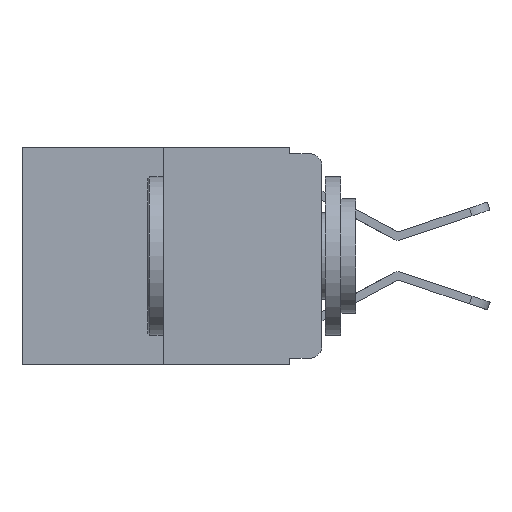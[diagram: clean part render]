
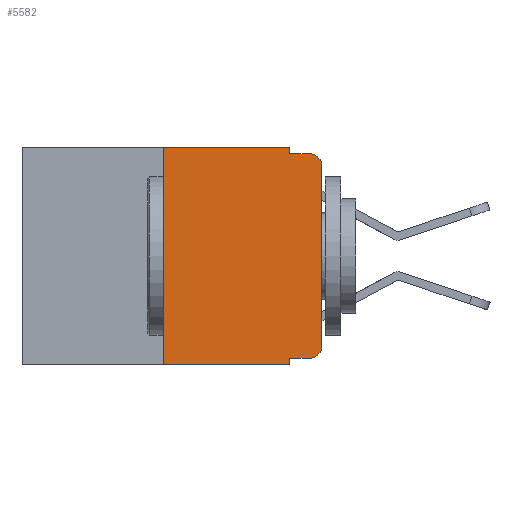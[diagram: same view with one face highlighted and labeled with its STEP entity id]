
A CAD part, left-side view. The second image highlights one B-rep face of the part: STEP entity #5582.
In plain terms, the highlighted planar face has unit normal (-1, 0, 0).
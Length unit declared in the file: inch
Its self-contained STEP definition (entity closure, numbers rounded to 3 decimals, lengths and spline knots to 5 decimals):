
#95 = VERTEX_POINT ( 'NONE', #556 ) ;
#371 = DIRECTION ( 'NONE',  ( 0., 0., 1. ) ) ;
#556 = CARTESIAN_POINT ( 'NONE',  ( 0., 0.051, -0.343 ) ) ;
#577 = EDGE_CURVE ( 'NONE', #708, #95, #7618, .T. ) ;
#708 = VERTEX_POINT ( 'NONE', #16838 ) ;
#1012 = LINE ( 'NONE', #12679, #2255 ) ;
#1242 = VERTEX_POINT ( 'NONE', #6102 ) ;
#1489 = VERTEX_POINT ( 'NONE', #12013 ) ;
#2255 = VECTOR ( 'NONE', #16822, 39.37008 ) ;
#2292 = EDGE_CURVE ( 'NONE', #1242, #5987, #1012, .T. ) ;
#2362 = EDGE_LOOP ( 'NONE', ( #12966, #10455, #10580, #13551, #6723, #7793, #7699, #6070, #3460, #5937 ) ) ;
#2534 = LINE ( 'NONE', #16949, #16936 ) ;
#2572 = DIRECTION ( 'NONE',  ( 0., -1., 0. ) ) ;
#3074 = VECTOR ( 'NONE', #4024, 39.37008 ) ;
#3460 = ORIENTED_EDGE ( 'NONE', *, *, #13911, .T. ) ;
#3461 = EDGE_CURVE ( 'NONE', #708, #11666, #15103, .T. ) ;
#4012 = DIRECTION ( 'NONE',  ( -1., 0., 0. ) ) ;
#4024 = DIRECTION ( 'NONE',  ( 0., 0., -1. ) ) ;
#4163 = DIRECTION ( 'NONE',  ( 0., -1., 0. ) ) ;
#4422 = CARTESIAN_POINT ( 'NONE',  ( 0., 0., 0. ) ) ;
#4485 = VERTEX_POINT ( 'NONE', #6245 ) ;
#4686 = EDGE_CURVE ( 'NONE', #11666, #1242, #9004, .T. ) ;
#5286 = DIRECTION ( 'NONE',  ( 1., 0., 0. ) ) ;
#5328 = CARTESIAN_POINT ( 'NONE',  ( 0., 0.02, -0.313 ) ) ;
#5380 = FACE_OUTER_BOUND ( 'NONE', #2362, .T. ) ;
#5458 = CARTESIAN_POINT ( 'NONE',  ( 0., 0.051, 0. ) ) ;
#5460 = PLANE ( 'NONE',  #8313 ) ;
#5499 = DIRECTION ( 'NONE',  ( 0., 0., -1. ) ) ;
#5582 = ADVANCED_FACE ( 'NONE', ( #5380 ), #5460, .F. ) ;
#5701 = LINE ( 'NONE', #7719, #11393 ) ;
#5756 = CARTESIAN_POINT ( 'NONE',  ( 0., 0.02, -0.01 ) ) ;
#5937 = ORIENTED_EDGE ( 'NONE', *, *, #6556, .T. ) ;
#5987 = VERTEX_POINT ( 'NONE', #14059 ) ;
#6070 = ORIENTED_EDGE ( 'NONE', *, *, #15875, .F. ) ;
#6102 = CARTESIAN_POINT ( 'NONE',  ( 0., 0.051, 0. ) ) ;
#6245 = CARTESIAN_POINT ( 'NONE',  ( 0., 0.02, -0.333 ) ) ;
#6556 = EDGE_CURVE ( 'NONE', #4485, #11104, #9183, .T. ) ;
#6686 = VECTOR ( 'NONE', #371, 39.37008 ) ;
#6723 = ORIENTED_EDGE ( 'NONE', *, *, #4686, .F. ) ;
#6859 = DIRECTION ( 'NONE',  ( -1., 0., 0. ) ) ;
#7618 = LINE ( 'NONE', #8434, #13956 ) ;
#7699 = ORIENTED_EDGE ( 'NONE', *, *, #577, .T. ) ;
#7719 = CARTESIAN_POINT ( 'NONE',  ( 0., 0.051, -0.333 ) ) ;
#7793 = ORIENTED_EDGE ( 'NONE', *, *, #3461, .F. ) ;
#7939 = VERTEX_POINT ( 'NONE', #5756 ) ;
#8172 = DIRECTION ( 'NONE',  ( 0., 0., -1. ) ) ;
#8313 = AXIS2_PLACEMENT_3D ( 'NONE', #9300, #5286, #8172 ) ;
#8434 = CARTESIAN_POINT ( 'NONE',  ( 0., 0.473, -0.343 ) ) ;
#9004 = LINE ( 'NONE', #10656, #13454 ) ;
#9183 = CIRCLE ( 'NONE', #13985, 0.02 ) ;
#9300 = CARTESIAN_POINT ( 'NONE',  ( 0., 0.473, 0. ) ) ;
#9343 = EDGE_CURVE ( 'NONE', #5987, #7939, #2534, .T. ) ;
#10279 = CARTESIAN_POINT ( 'NONE',  ( 0., 0.25, 0. ) ) ;
#10343 = DIRECTION ( 'NONE',  ( 0., -1., 0. ) ) ;
#10455 = ORIENTED_EDGE ( 'NONE', *, *, #16005, .T. ) ;
#10580 = ORIENTED_EDGE ( 'NONE', *, *, #9343, .F. ) ;
#10656 = CARTESIAN_POINT ( 'NONE',  ( 0., 0.473, 0. ) ) ;
#10999 = DIRECTION ( 'NONE',  ( 0., 0., -1. ) ) ;
#11104 = VERTEX_POINT ( 'NONE', #11302 ) ;
#11227 = CARTESIAN_POINT ( 'NONE',  ( 0., 0.25, 0. ) ) ;
#11302 = CARTESIAN_POINT ( 'NONE',  ( 0., 0., -0.313 ) ) ;
#11393 = VECTOR ( 'NONE', #2572, 39.37008 ) ;
#11666 = VERTEX_POINT ( 'NONE', #11227 ) ;
#11704 = VECTOR ( 'NONE', #13081, 39.37008 ) ;
#12013 = CARTESIAN_POINT ( 'NONE',  ( 0., 0., -0.03 ) ) ;
#12679 = CARTESIAN_POINT ( 'NONE',  ( 0., 0.051, 0. ) ) ;
#12704 = VERTEX_POINT ( 'NONE', #14508 ) ;
#12853 = AXIS2_PLACEMENT_3D ( 'NONE', #13725, #6859, #10999 ) ;
#12966 = ORIENTED_EDGE ( 'NONE', *, *, #16520, .T. ) ;
#13081 = DIRECTION ( 'NONE',  ( 0., 0., 1. ) ) ;
#13454 = VECTOR ( 'NONE', #14627, 39.37008 ) ;
#13551 = ORIENTED_EDGE ( 'NONE', *, *, #2292, .F. ) ;
#13725 = CARTESIAN_POINT ( 'NONE',  ( 0., 0.02, -0.03 ) ) ;
#13911 = EDGE_CURVE ( 'NONE', #12704, #4485, #5701, .T. ) ;
#13956 = VECTOR ( 'NONE', #4163, 39.37008 ) ;
#13985 = AXIS2_PLACEMENT_3D ( 'NONE', #5328, #4012, #5499 ) ;
#14059 = CARTESIAN_POINT ( 'NONE',  ( 0., 0.051, -0.01 ) ) ;
#14508 = CARTESIAN_POINT ( 'NONE',  ( 0., 0.051, -0.333 ) ) ;
#14627 = DIRECTION ( 'NONE',  ( 0., -1., 0. ) ) ;
#14727 = LINE ( 'NONE', #4422, #6686 ) ;
#15103 = LINE ( 'NONE', #10279, #11704 ) ;
#15875 = EDGE_CURVE ( 'NONE', #12704, #95, #16222, .T. ) ;
#16005 = EDGE_CURVE ( 'NONE', #1489, #7939, #16679, .T. ) ;
#16222 = LINE ( 'NONE', #5458, #3074 ) ;
#16520 = EDGE_CURVE ( 'NONE', #11104, #1489, #14727, .T. ) ;
#16679 = CIRCLE ( 'NONE', #12853, 0.02 ) ;
#16822 = DIRECTION ( 'NONE',  ( 0., 0., -1. ) ) ;
#16838 = CARTESIAN_POINT ( 'NONE',  ( 0., 0.25, -0.343 ) ) ;
#16936 = VECTOR ( 'NONE', #10343, 39.37008 ) ;
#16949 = CARTESIAN_POINT ( 'NONE',  ( 0., 0.051, -0.01 ) ) ;
